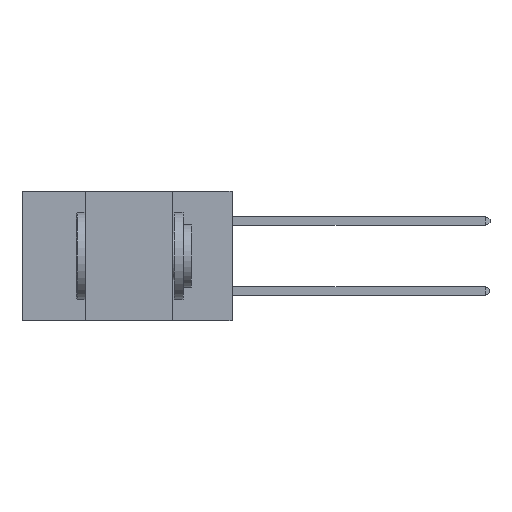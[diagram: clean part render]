
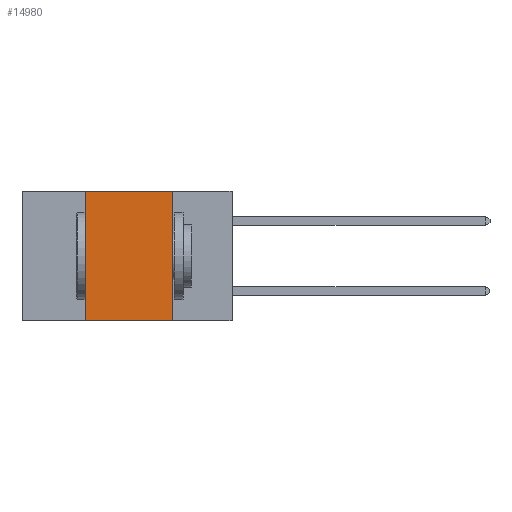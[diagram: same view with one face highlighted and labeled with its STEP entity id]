
A CAD part, left-side view. The second image highlights one B-rep face of the part: STEP entity #14980.
In plain terms, the highlighted planar face has unit normal (-1, 0, 0).
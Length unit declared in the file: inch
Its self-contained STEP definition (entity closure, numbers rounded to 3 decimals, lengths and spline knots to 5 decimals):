
#25 = CARTESIAN_POINT ( 'NONE',  ( 0., 0.6, 0. ) ) ;
#249 = CARTESIAN_POINT ( 'NONE',  ( 0., 0.42, 0. ) ) ;
#280 = DIRECTION ( 'NONE',  ( 0., 0., 1. ) ) ;
#341 = DIRECTION ( 'NONE',  ( 0., 0., -1. ) ) ;
#460 = EDGE_CURVE ( 'NONE', #11657, #2950, #11704, .T. ) ;
#1835 = ORIENTED_EDGE ( 'NONE', *, *, #3591, .F. ) ;
#2173 = VECTOR ( 'NONE', #4843, 39.37008 ) ;
#2433 = PLANE ( 'NONE',  #12950 ) ;
#2950 = VERTEX_POINT ( 'NONE', #6403 ) ;
#3214 = VECTOR ( 'NONE', #280, 39.37008 ) ;
#3591 = EDGE_CURVE ( 'NONE', #10911, #11657, #9950, .T. ) ;
#3643 = DIRECTION ( 'NONE',  ( 0., 0., -1. ) ) ;
#4116 = VECTOR ( 'NONE', #341, 39.37008 ) ;
#4223 = FACE_OUTER_BOUND ( 'NONE', #10801, .T. ) ;
#4278 = ORIENTED_EDGE ( 'NONE', *, *, #8932, .F. ) ;
#4547 = CARTESIAN_POINT ( 'NONE',  ( 0., 0.6, 0. ) ) ;
#4843 = DIRECTION ( 'NONE',  ( 0., -1., 0. ) ) ;
#5070 = VECTOR ( 'NONE', #8141, 39.37008 ) ;
#6294 = CARTESIAN_POINT ( 'NONE',  ( 0., 0.17, 0. ) ) ;
#6403 = CARTESIAN_POINT ( 'NONE',  ( 0., 0.17, 0. ) ) ;
#6855 = CARTESIAN_POINT ( 'NONE',  ( 0., 0.17, -0.37 ) ) ;
#7547 = CARTESIAN_POINT ( 'NONE',  ( 0., 0.42, -0.37 ) ) ;
#7715 = VERTEX_POINT ( 'NONE', #6855 ) ;
#7760 = EDGE_CURVE ( 'NONE', #10911, #7715, #8608, .T. ) ;
#8141 = DIRECTION ( 'NONE',  ( 0., -1., 0. ) ) ;
#8608 = LINE ( 'NONE', #14051, #5070 ) ;
#8932 = EDGE_CURVE ( 'NONE', #2950, #7715, #10474, .T. ) ;
#9563 = CARTESIAN_POINT ( 'NONE',  ( 0., 0.42, 0. ) ) ;
#9950 = LINE ( 'NONE', #249, #3214 ) ;
#10185 = ORIENTED_EDGE ( 'NONE', *, *, #7760, .T. ) ;
#10474 = LINE ( 'NONE', #6294, #4116 ) ;
#10801 = EDGE_LOOP ( 'NONE', ( #4278, #15007, #1835, #10185 ) ) ;
#10805 = DIRECTION ( 'NONE',  ( 1., 0., 0. ) ) ;
#10911 = VERTEX_POINT ( 'NONE', #7547 ) ;
#11657 = VERTEX_POINT ( 'NONE', #9563 ) ;
#11704 = LINE ( 'NONE', #4547, #2173 ) ;
#12950 = AXIS2_PLACEMENT_3D ( 'NONE', #25, #10805, #3643 ) ;
#14051 = CARTESIAN_POINT ( 'NONE',  ( 0., 0.6, -0.37 ) ) ;
#14980 = ADVANCED_FACE ( 'NONE', ( #4223 ), #2433, .F. ) ;
#15007 = ORIENTED_EDGE ( 'NONE', *, *, #460, .F. ) ;
